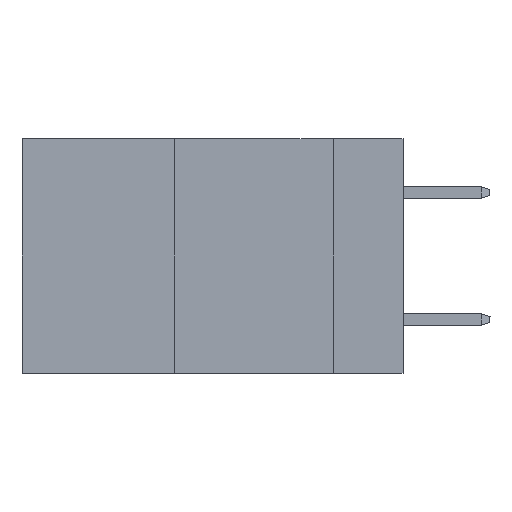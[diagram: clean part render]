
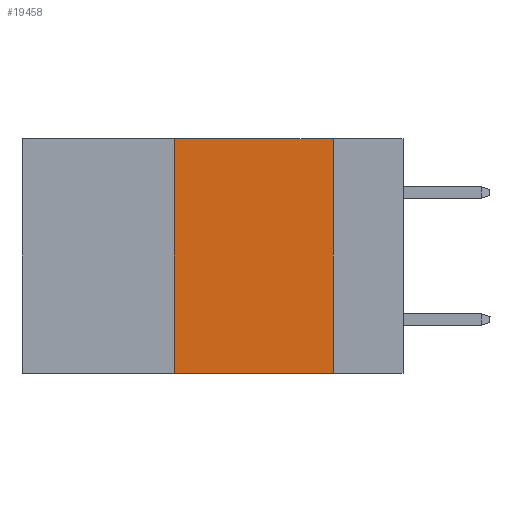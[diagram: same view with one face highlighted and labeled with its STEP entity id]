
A CAD part, left-side view. The second image highlights one B-rep face of the part: STEP entity #19458.
In plain terms, the highlighted planar face has unit normal (-1, 0, 0).
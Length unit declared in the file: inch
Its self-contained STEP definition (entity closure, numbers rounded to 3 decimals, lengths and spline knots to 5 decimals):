
#328 = DIRECTION ( 'NONE',  ( 1., 0., 0. ) ) ;
#1149 = CARTESIAN_POINT ( 'NONE',  ( 0., 0.36, -0.37 ) ) ;
#1490 = LINE ( 'NONE', #20152, #7812 ) ;
#2206 = EDGE_CURVE ( 'NONE', #11372, #9118, #1490, .T. ) ;
#2694 = EDGE_CURVE ( 'NONE', #10348, #21688, #15814, .T. ) ;
#4261 = LINE ( 'NONE', #14128, #17960 ) ;
#5566 = ORIENTED_EDGE ( 'NONE', *, *, #22023, .T. ) ;
#5848 = ORIENTED_EDGE ( 'NONE', *, *, #2694, .F. ) ;
#6270 = DIRECTION ( 'NONE',  ( 0., 0., 1. ) ) ;
#6706 = CARTESIAN_POINT ( 'NONE',  ( 0., 0.6, 0. ) ) ;
#7812 = VECTOR ( 'NONE', #17260, 39.37008 ) ;
#9089 = DIRECTION ( 'NONE',  ( 0., 0., -1. ) ) ;
#9118 = VERTEX_POINT ( 'NONE', #26459 ) ;
#9394 = FACE_OUTER_BOUND ( 'NONE', #28854, .T. ) ;
#10348 = VERTEX_POINT ( 'NONE', #1149 ) ;
#11034 = AXIS2_PLACEMENT_3D ( 'NONE', #6706, #328, #9089 ) ;
#11372 = VERTEX_POINT ( 'NONE', #15187 ) ;
#11522 = PLANE ( 'NONE',  #11034 ) ;
#12497 = CARTESIAN_POINT ( 'NONE',  ( 0., 0.36, 0. ) ) ;
#14128 = CARTESIAN_POINT ( 'NONE',  ( 0., 0.6, -0.37 ) ) ;
#14496 = CARTESIAN_POINT ( 'NONE',  ( 0., 0.6, 0. ) ) ;
#15187 = CARTESIAN_POINT ( 'NONE',  ( 0., 0.11, 0. ) ) ;
#15814 = LINE ( 'NONE', #25053, #18024 ) ;
#17260 = DIRECTION ( 'NONE',  ( 0., 0., -1. ) ) ;
#17960 = VECTOR ( 'NONE', #18689, 39.37008 ) ;
#18024 = VECTOR ( 'NONE', #6270, 39.37008 ) ;
#18689 = DIRECTION ( 'NONE',  ( 0., -1., 0. ) ) ;
#19458 = ADVANCED_FACE ( 'NONE', ( #9394 ), #11522, .F. ) ;
#19983 = EDGE_CURVE ( 'NONE', #21688, #11372, #28137, .T. ) ;
#20152 = CARTESIAN_POINT ( 'NONE',  ( 0., 0.11, 0. ) ) ;
#21688 = VERTEX_POINT ( 'NONE', #12497 ) ;
#22023 = EDGE_CURVE ( 'NONE', #10348, #9118, #4261, .T. ) ;
#23311 = DIRECTION ( 'NONE',  ( 0., -1., 0. ) ) ;
#25053 = CARTESIAN_POINT ( 'NONE',  ( 0., 0.36, 0. ) ) ;
#26459 = CARTESIAN_POINT ( 'NONE',  ( 0., 0.11, -0.37 ) ) ;
#26816 = ORIENTED_EDGE ( 'NONE', *, *, #19983, .F. ) ;
#28137 = LINE ( 'NONE', #14496, #29443 ) ;
#28854 = EDGE_LOOP ( 'NONE', ( #29767, #26816, #5848, #5566 ) ) ;
#29443 = VECTOR ( 'NONE', #23311, 39.37008 ) ;
#29767 = ORIENTED_EDGE ( 'NONE', *, *, #2206, .F. ) ;
